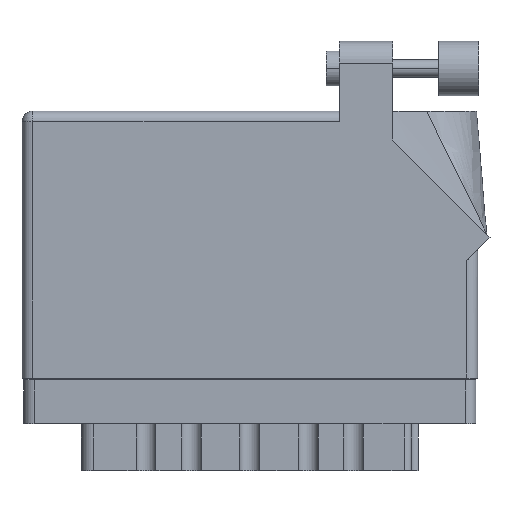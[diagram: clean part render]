
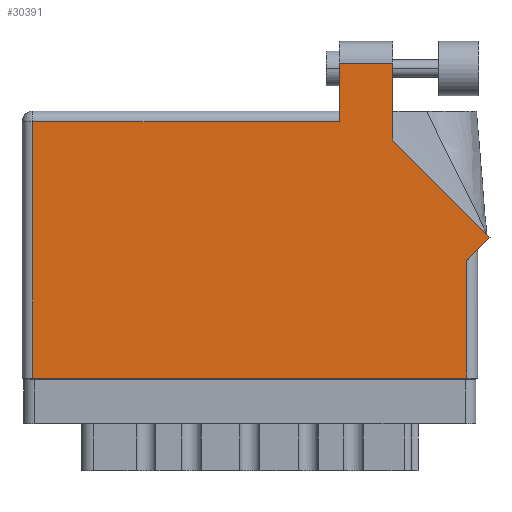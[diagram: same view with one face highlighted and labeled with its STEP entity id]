
A CAD part, front view. The second image highlights one B-rep face of the part: STEP entity #30391.
In plain terms, the highlighted face is planar.
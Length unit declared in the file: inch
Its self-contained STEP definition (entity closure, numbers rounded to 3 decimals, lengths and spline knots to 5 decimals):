
#820 = VECTOR ( 'NONE', #19641, 39.37008 ) ;
#845 = LINE ( 'NONE', #23867, #4874 ) ;
#2146 = VERTEX_POINT ( 'NONE', #25863 ) ;
#2616 = VECTOR ( 'NONE', #21283, 39.37008 ) ;
#3370 = CARTESIAN_POINT ( 'NONE',  ( 2.68271, 0.80771, 0. ) ) ;
#3581 = VERTEX_POINT ( 'NONE', #32950 ) ;
#4874 = VECTOR ( 'NONE', #16112, 39.37008 ) ;
#5554 = LINE ( 'NONE', #12315, #37658 ) ;
#5719 = EDGE_CURVE ( 'NONE', #34782, #48747, #22538, .T. ) ;
#5972 = VECTOR ( 'NONE', #42137, 39.37008 ) ;
#6496 = DIRECTION ( 'NONE',  ( 0., 1., 0. ) ) ;
#7232 = CARTESIAN_POINT ( 'NONE',  ( 2.55, 0.737, 0. ) ) ;
#10267 = ORIENTED_EDGE ( 'NONE', *, *, #41731, .T. ) ;
#10445 = ORIENTED_EDGE ( 'NONE', *, *, #48593, .T. ) ;
#10823 = CARTESIAN_POINT ( 'NONE',  ( 2.612, 0.737, 0. ) ) ;
#11212 = VERTEX_POINT ( 'NONE', #24553 ) ;
#11796 = DIRECTION ( 'NONE',  ( 0., 0., -1. ) ) ;
#12202 = VERTEX_POINT ( 'NONE', #3370 ) ;
#12315 = CARTESIAN_POINT ( 'NONE',  ( 0.062, 0., 0. ) ) ;
#14087 = LINE ( 'NONE', #10823, #31964 ) ;
#14554 = VECTOR ( 'NONE', #48638, 39.37008 ) ;
#15575 = CARTESIAN_POINT ( 'NONE',  ( 1.819, 1.468, 0. ) ) ;
#16112 = DIRECTION ( 'NONE',  ( -0.707, 0.707, 0. ) ) ;
#16427 = VERTEX_POINT ( 'NONE', #43160 ) ;
#17554 = ORIENTED_EDGE ( 'NONE', *, *, #49543, .T. ) ;
#19641 = DIRECTION ( 'NONE',  ( -1., 0., 0. ) ) ;
#19755 = AXIS2_PLACEMENT_3D ( 'NONE', #41389, #11796, #42386 ) ;
#19789 = DIRECTION ( 'NONE',  ( 1., 0., 0. ) ) ;
#21283 = DIRECTION ( 'NONE',  ( -1., 0., 0. ) ) ;
#21533 = EDGE_CURVE ( 'NONE', #3581, #32390, #5554, .T. ) ;
#22538 = LINE ( 'NONE', #30562, #14554 ) ;
#22670 = EDGE_CURVE ( 'NONE', #12202, #16427, #845, .T. ) ;
#23534 = ORIENTED_EDGE ( 'NONE', *, *, #22670, .T. ) ;
#23867 = CARTESIAN_POINT ( 'NONE',  ( 2.68271, 0.80771, 0. ) ) ;
#24287 = CARTESIAN_POINT ( 'NONE',  ( 0., 0., 0. ) ) ;
#24553 = CARTESIAN_POINT ( 'NONE',  ( 2.55, 0., 0. ) ) ;
#25018 = LINE ( 'NONE', #41320, #2616 ) ;
#25863 = CARTESIAN_POINT ( 'NONE',  ( 2.126, 1.805, 0. ) ) ;
#26089 = DIRECTION ( 'NONE',  ( 0.707, 0.707, 0. ) ) ;
#26252 = LINE ( 'NONE', #7232, #42217 ) ;
#27061 = PLANE ( 'NONE',  #19755 ) ;
#27377 = EDGE_LOOP ( 'NONE', ( #10267, #17554, #29882, #40019, #39679, #38237, #41915, #10445, #23534 ) ) ;
#29882 = ORIENTED_EDGE ( 'NONE', *, *, #5719, .T. ) ;
#30391 = ADVANCED_FACE ( 'NONE', ( #45910 ), #27061, .F. ) ;
#30562 = CARTESIAN_POINT ( 'NONE',  ( 1.819, 1.53, 0. ) ) ;
#31964 = VECTOR ( 'NONE', #26089, 39.37008 ) ;
#32390 = VERTEX_POINT ( 'NONE', #42133 ) ;
#32950 = CARTESIAN_POINT ( 'NONE',  ( 0.062, 1.468, 0. ) ) ;
#33388 = CARTESIAN_POINT ( 'NONE',  ( 2.55, 0.675, 0. ) ) ;
#33943 = VECTOR ( 'NONE', #19789, 39.37008 ) ;
#34782 = VERTEX_POINT ( 'NONE', #48974 ) ;
#35720 = VERTEX_POINT ( 'NONE', #33388 ) ;
#35824 = LINE ( 'NONE', #24287, #33943 ) ;
#36023 = LINE ( 'NONE', #45903, #5972 ) ;
#37658 = VECTOR ( 'NONE', #42913, 39.37008 ) ;
#37712 = EDGE_CURVE ( 'NONE', #32390, #11212, #35824, .T. ) ;
#38237 = ORIENTED_EDGE ( 'NONE', *, *, #37712, .T. ) ;
#38710 = LINE ( 'NONE', #42975, #820 ) ;
#39679 = ORIENTED_EDGE ( 'NONE', *, *, #21533, .T. ) ;
#40019 = ORIENTED_EDGE ( 'NONE', *, *, #40244, .T. ) ;
#40244 = EDGE_CURVE ( 'NONE', #48747, #3581, #25018, .T. ) ;
#41320 = CARTESIAN_POINT ( 'NONE',  ( 0., 1.468, 0. ) ) ;
#41389 = CARTESIAN_POINT ( 'NONE',  ( 0., 1.53, 0. ) ) ;
#41731 = EDGE_CURVE ( 'NONE', #16427, #2146, #36023, .T. ) ;
#41915 = ORIENTED_EDGE ( 'NONE', *, *, #46803, .T. ) ;
#42133 = CARTESIAN_POINT ( 'NONE',  ( 0.062, 0., 0. ) ) ;
#42137 = DIRECTION ( 'NONE',  ( 0., 1., 0. ) ) ;
#42217 = VECTOR ( 'NONE', #6496, 39.37008 ) ;
#42386 = DIRECTION ( 'NONE',  ( -1., 0., 0. ) ) ;
#42913 = DIRECTION ( 'NONE',  ( 0., -1., 0. ) ) ;
#42975 = CARTESIAN_POINT ( 'NONE',  ( 1.819, 1.805, 0. ) ) ;
#43160 = CARTESIAN_POINT ( 'NONE',  ( 2.126, 1.36442, 0. ) ) ;
#45903 = CARTESIAN_POINT ( 'NONE',  ( 2.126, 1.36442, 0. ) ) ;
#45910 = FACE_OUTER_BOUND ( 'NONE', #27377, .T. ) ;
#46803 = EDGE_CURVE ( 'NONE', #11212, #35720, #26252, .T. ) ;
#48593 = EDGE_CURVE ( 'NONE', #35720, #12202, #14087, .T. ) ;
#48638 = DIRECTION ( 'NONE',  ( 0., -1., 0. ) ) ;
#48747 = VERTEX_POINT ( 'NONE', #15575 ) ;
#48974 = CARTESIAN_POINT ( 'NONE',  ( 1.819, 1.805, 0. ) ) ;
#49543 = EDGE_CURVE ( 'NONE', #2146, #34782, #38710, .T. ) ;
